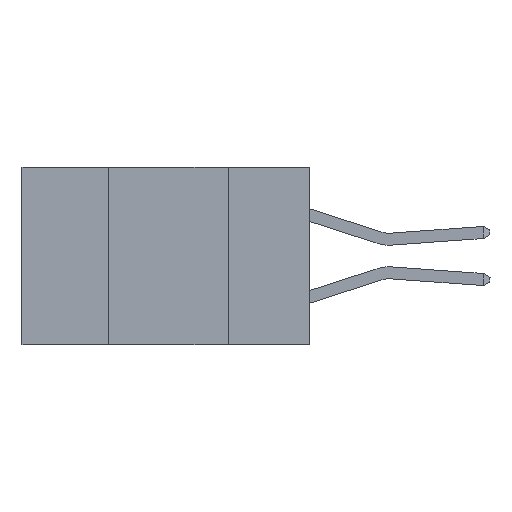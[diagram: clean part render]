
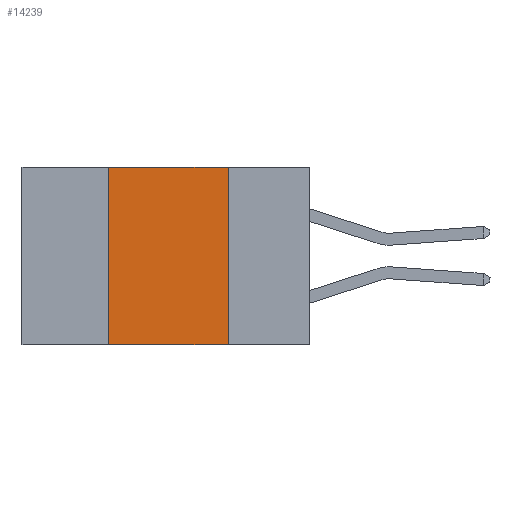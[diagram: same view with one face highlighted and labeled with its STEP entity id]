
A CAD part, left-side view. The second image highlights one B-rep face of the part: STEP entity #14239.
In plain terms, the highlighted planar face has unit normal (-1, 0, 0).
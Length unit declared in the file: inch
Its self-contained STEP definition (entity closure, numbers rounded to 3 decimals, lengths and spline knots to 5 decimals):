
#205 = LINE ( 'NONE', #2107, #3931 ) ;
#703 = VECTOR ( 'NONE', #9083, 39.37008 ) ;
#2107 = CARTESIAN_POINT ( 'NONE',  ( 0., 0.17, 0. ) ) ;
#2336 = VERTEX_POINT ( 'NONE', #10522 ) ;
#2427 = EDGE_CURVE ( 'NONE', #11931, #3828, #205, .T. ) ;
#2785 = LINE ( 'NONE', #13403, #11408 ) ;
#3713 = EDGE_CURVE ( 'NONE', #5622, #3828, #12870, .T. ) ;
#3828 = VERTEX_POINT ( 'NONE', #12181 ) ;
#3931 = VECTOR ( 'NONE', #4327, 39.37008 ) ;
#4019 = CARTESIAN_POINT ( 'NONE',  ( 0., 0.6, 0. ) ) ;
#4327 = DIRECTION ( 'NONE',  ( 0., 0., -1. ) ) ;
#4657 = CARTESIAN_POINT ( 'NONE',  ( 0., 0.6, -0.37 ) ) ;
#5196 = PLANE ( 'NONE',  #9365 ) ;
#5238 = ORIENTED_EDGE ( 'NONE', *, *, #2427, .F. ) ;
#5286 = DIRECTION ( 'NONE',  ( 1., 0., 0. ) ) ;
#5343 = FACE_OUTER_BOUND ( 'NONE', #8545, .T. ) ;
#5622 = VERTEX_POINT ( 'NONE', #12928 ) ;
#5988 = CARTESIAN_POINT ( 'NONE',  ( 0., 0.17, 0. ) ) ;
#6416 = EDGE_CURVE ( 'NONE', #2336, #11931, #8610, .T. ) ;
#8545 = EDGE_LOOP ( 'NONE', ( #5238, #11632, #13820, #14014 ) ) ;
#8610 = LINE ( 'NONE', #4019, #11207 ) ;
#9083 = DIRECTION ( 'NONE',  ( 0., -1., 0. ) ) ;
#9365 = AXIS2_PLACEMENT_3D ( 'NONE', #10711, #5286, #14299 ) ;
#10522 = CARTESIAN_POINT ( 'NONE',  ( 0., 0.42, 0. ) ) ;
#10711 = CARTESIAN_POINT ( 'NONE',  ( 0., 0.6, 0. ) ) ;
#10720 = DIRECTION ( 'NONE',  ( 0., -1., 0. ) ) ;
#10909 = EDGE_CURVE ( 'NONE', #5622, #2336, #2785, .T. ) ;
#11123 = DIRECTION ( 'NONE',  ( 0., 0., 1. ) ) ;
#11207 = VECTOR ( 'NONE', #10720, 39.37008 ) ;
#11408 = VECTOR ( 'NONE', #11123, 39.37008 ) ;
#11632 = ORIENTED_EDGE ( 'NONE', *, *, #6416, .F. ) ;
#11931 = VERTEX_POINT ( 'NONE', #5988 ) ;
#12181 = CARTESIAN_POINT ( 'NONE',  ( 0., 0.17, -0.37 ) ) ;
#12870 = LINE ( 'NONE', #4657, #703 ) ;
#12928 = CARTESIAN_POINT ( 'NONE',  ( 0., 0.42, -0.37 ) ) ;
#13403 = CARTESIAN_POINT ( 'NONE',  ( 0., 0.42, 0. ) ) ;
#13820 = ORIENTED_EDGE ( 'NONE', *, *, #10909, .F. ) ;
#14014 = ORIENTED_EDGE ( 'NONE', *, *, #3713, .T. ) ;
#14239 = ADVANCED_FACE ( 'NONE', ( #5343 ), #5196, .F. ) ;
#14299 = DIRECTION ( 'NONE',  ( 0., 0., -1. ) ) ;
